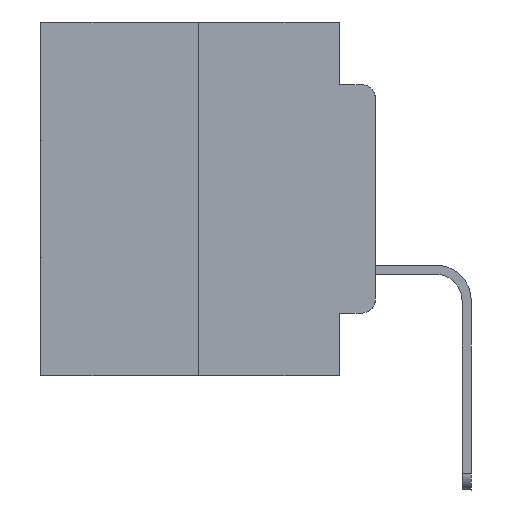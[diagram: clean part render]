
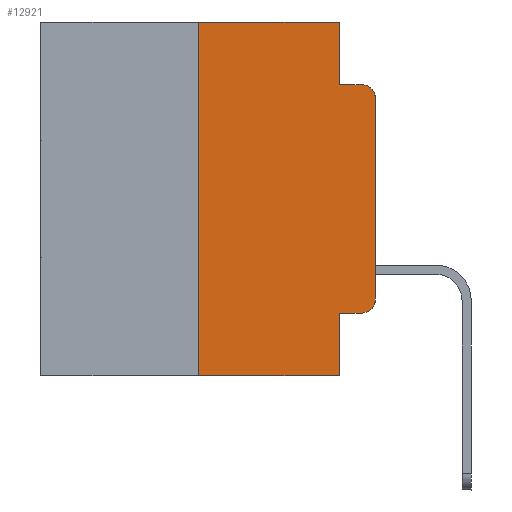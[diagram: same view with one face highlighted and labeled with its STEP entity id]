
A CAD part, left-side view. The second image highlights one B-rep face of the part: STEP entity #12921.
In plain terms, the highlighted planar face has unit normal (-1, 0, 0).
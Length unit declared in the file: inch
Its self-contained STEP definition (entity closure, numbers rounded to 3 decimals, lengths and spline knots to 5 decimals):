
#656 = LINE ( 'NONE', #20121, #11251 ) ;
#743 = VERTEX_POINT ( 'NONE', #12154 ) ;
#1666 = CARTESIAN_POINT ( 'NONE',  ( 0., 0.051, -0.4115 ) ) ;
#1967 = CARTESIAN_POINT ( 'NONE',  ( 0., 0.051, -0.4115 ) ) ;
#2449 = CARTESIAN_POINT ( 'NONE',  ( 0., 0.473, 0. ) ) ;
#2580 = ORIENTED_EDGE ( 'NONE', *, *, #24793, .T. ) ;
#2903 = VERTEX_POINT ( 'NONE', #1666 ) ;
#3350 = LINE ( 'NONE', #13094, #12984 ) ;
#3938 = EDGE_CURVE ( 'NONE', #8703, #20215, #3350, .T. ) ;
#4065 = CARTESIAN_POINT ( 'NONE',  ( 0., 0., 0. ) ) ;
#5030 = AXIS2_PLACEMENT_3D ( 'NONE', #18395, #12486, #6153 ) ;
#5131 = CARTESIAN_POINT ( 'NONE',  ( 0., 0., -0.1085 ) ) ;
#5706 = EDGE_CURVE ( 'NONE', #21314, #743, #23519, .T. ) ;
#6033 = DIRECTION ( 'NONE',  ( 0., -1., 0. ) ) ;
#6153 = DIRECTION ( 'NONE',  ( 0., 0., -1. ) ) ;
#6204 = CIRCLE ( 'NONE', #8122, 0.02 ) ;
#6215 = AXIS2_PLACEMENT_3D ( 'NONE', #2449, #16794, #6606 ) ;
#6606 = DIRECTION ( 'NONE',  ( 0., 0., -1. ) ) ;
#6716 = ORIENTED_EDGE ( 'NONE', *, *, #5706, .T. ) ;
#6923 = VECTOR ( 'NONE', #15512, 39.37008 ) ;
#7067 = DIRECTION ( 'NONE',  ( 0., -1., 0. ) ) ;
#7143 = VERTEX_POINT ( 'NONE', #5131 ) ;
#7251 = ORIENTED_EDGE ( 'NONE', *, *, #24502, .T. ) ;
#7351 = ORIENTED_EDGE ( 'NONE', *, *, #15672, .T. ) ;
#7463 = LINE ( 'NONE', #1967, #16418 ) ;
#7683 = VERTEX_POINT ( 'NONE', #26353 ) ;
#8122 = AXIS2_PLACEMENT_3D ( 'NONE', #13118, #11304, #11046 ) ;
#8391 = CARTESIAN_POINT ( 'NONE',  ( 0., 0.051, -0.0885 ) ) ;
#8703 = VERTEX_POINT ( 'NONE', #12682 ) ;
#9158 = EDGE_CURVE ( 'NONE', #2903, #743, #9587, .T. ) ;
#9370 = CARTESIAN_POINT ( 'NONE',  ( 0., 0.25, -0.5 ) ) ;
#9528 = ORIENTED_EDGE ( 'NONE', *, *, #3938, .F. ) ;
#9587 = LINE ( 'NONE', #13668, #16326 ) ;
#10276 = CARTESIAN_POINT ( 'NONE',  ( 0., 0.051, -0.0885 ) ) ;
#11046 = DIRECTION ( 'NONE',  ( 0., 0., -1. ) ) ;
#11251 = VECTOR ( 'NONE', #11909, 39.37008 ) ;
#11304 = DIRECTION ( 'NONE',  ( -1., 0., 0. ) ) ;
#11354 = ORIENTED_EDGE ( 'NONE', *, *, #15528, .F. ) ;
#11909 = DIRECTION ( 'NONE',  ( 0., 0., 1. ) ) ;
#12154 = CARTESIAN_POINT ( 'NONE',  ( 0., 0.051, -0.5 ) ) ;
#12206 = DIRECTION ( 'NONE',  ( 0., 0., 1. ) ) ;
#12486 = DIRECTION ( 'NONE',  ( -1., 0., 0. ) ) ;
#12663 = PLANE ( 'NONE',  #6215 ) ;
#12682 = CARTESIAN_POINT ( 'NONE',  ( 0., 0.051, 0. ) ) ;
#12921 = ADVANCED_FACE ( 'NONE', ( #25561 ), #12663, .F. ) ;
#12984 = VECTOR ( 'NONE', #21458, 39.37008 ) ;
#13094 = CARTESIAN_POINT ( 'NONE',  ( 0., 0.051, 0. ) ) ;
#13118 = CARTESIAN_POINT ( 'NONE',  ( 0., 0.02, -0.1085 ) ) ;
#13424 = EDGE_LOOP ( 'NONE', ( #7351, #7251, #20693, #9528, #11354, #17242, #6716, #14310, #2580, #21979 ) ) ;
#13544 = CARTESIAN_POINT ( 'NONE',  ( 0., 0.473, -0.5 ) ) ;
#13668 = CARTESIAN_POINT ( 'NONE',  ( 0., 0.051, 0. ) ) ;
#13830 = VERTEX_POINT ( 'NONE', #22063 ) ;
#14310 = ORIENTED_EDGE ( 'NONE', *, *, #9158, .F. ) ;
#15455 = LINE ( 'NONE', #4065, #18958 ) ;
#15512 = DIRECTION ( 'NONE',  ( 0., -1., 0. ) ) ;
#15528 = EDGE_CURVE ( 'NONE', #21797, #8703, #17079, .T. ) ;
#15672 = EDGE_CURVE ( 'NONE', #13830, #7143, #15455, .T. ) ;
#16175 = EDGE_CURVE ( 'NONE', #21314, #21797, #656, .T. ) ;
#16326 = VECTOR ( 'NONE', #24291, 39.37008 ) ;
#16418 = VECTOR ( 'NONE', #6033, 39.37008 ) ;
#16700 = CARTESIAN_POINT ( 'NONE',  ( 0., 0.25, 0. ) ) ;
#16794 = DIRECTION ( 'NONE',  ( 1., 0., 0. ) ) ;
#17079 = LINE ( 'NONE', #23921, #18647 ) ;
#17242 = ORIENTED_EDGE ( 'NONE', *, *, #16175, .F. ) ;
#18042 = LINE ( 'NONE', #8391, #18994 ) ;
#18395 = CARTESIAN_POINT ( 'NONE',  ( 0., 0.02, -0.3915 ) ) ;
#18647 = VECTOR ( 'NONE', #7067, 39.37008 ) ;
#18958 = VECTOR ( 'NONE', #12206, 39.37008 ) ;
#18994 = VECTOR ( 'NONE', #22686, 39.37008 ) ;
#20121 = CARTESIAN_POINT ( 'NONE',  ( 0., 0.25, 0. ) ) ;
#20215 = VERTEX_POINT ( 'NONE', #10276 ) ;
#20693 = ORIENTED_EDGE ( 'NONE', *, *, #22963, .F. ) ;
#21314 = VERTEX_POINT ( 'NONE', #9370 ) ;
#21458 = DIRECTION ( 'NONE',  ( 0., 0., -1. ) ) ;
#21537 = CIRCLE ( 'NONE', #5030, 0.02 ) ;
#21797 = VERTEX_POINT ( 'NONE', #16700 ) ;
#21979 = ORIENTED_EDGE ( 'NONE', *, *, #24306, .T. ) ;
#22063 = CARTESIAN_POINT ( 'NONE',  ( 0., 0., -0.3915 ) ) ;
#22228 = VERTEX_POINT ( 'NONE', #22814 ) ;
#22686 = DIRECTION ( 'NONE',  ( 0., -1., 0. ) ) ;
#22814 = CARTESIAN_POINT ( 'NONE',  ( 0., 0.02, -0.4115 ) ) ;
#22963 = EDGE_CURVE ( 'NONE', #20215, #7683, #18042, .T. ) ;
#23519 = LINE ( 'NONE', #13544, #6923 ) ;
#23921 = CARTESIAN_POINT ( 'NONE',  ( 0., 0.473, 0. ) ) ;
#24291 = DIRECTION ( 'NONE',  ( 0., 0., -1. ) ) ;
#24306 = EDGE_CURVE ( 'NONE', #22228, #13830, #21537, .T. ) ;
#24502 = EDGE_CURVE ( 'NONE', #7143, #7683, #6204, .T. ) ;
#24793 = EDGE_CURVE ( 'NONE', #2903, #22228, #7463, .T. ) ;
#25561 = FACE_OUTER_BOUND ( 'NONE', #13424, .T. ) ;
#26353 = CARTESIAN_POINT ( 'NONE',  ( 0., 0.02, -0.0885 ) ) ;
